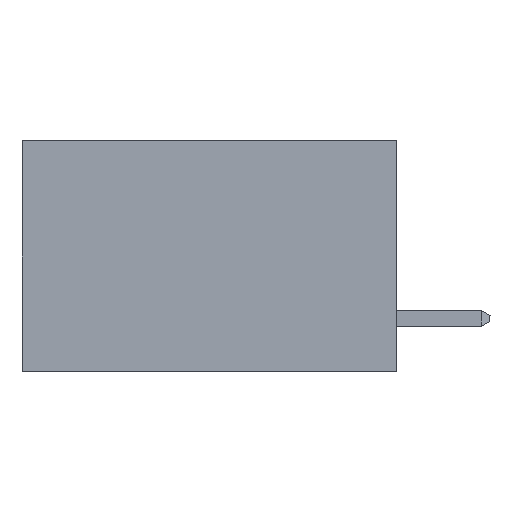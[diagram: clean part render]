
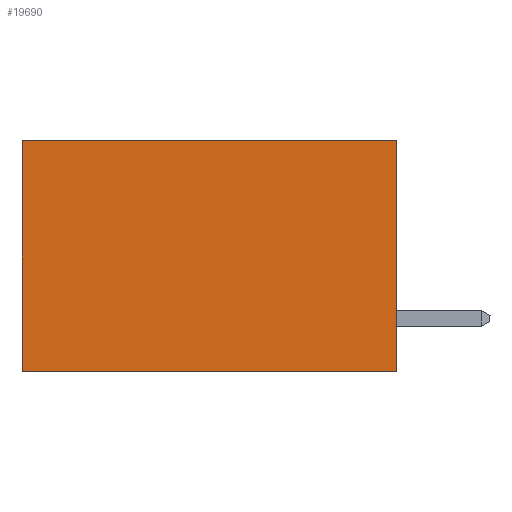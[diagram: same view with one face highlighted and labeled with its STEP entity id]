
A CAD part, left-side view. The second image highlights one B-rep face of the part: STEP entity #19690.
In plain terms, the highlighted planar face has unit normal (-1, 0, 0).
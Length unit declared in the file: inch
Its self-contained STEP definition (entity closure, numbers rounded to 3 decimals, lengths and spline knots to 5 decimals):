
#173 = DIRECTION ( 'NONE',  ( 0., 0., -1. ) ) ;
#183 = LINE ( 'NONE', #4333, #14905 ) ;
#1043 = CARTESIAN_POINT ( 'NONE',  ( 0.2615, 0.6, -0.37 ) ) ;
#1919 = ORIENTED_EDGE ( 'NONE', *, *, #18246, .T. ) ;
#2238 = AXIS2_PLACEMENT_3D ( 'NONE', #3078, #10826, #23860 ) ;
#2930 = VECTOR ( 'NONE', #15390, 39.37008 ) ;
#3078 = CARTESIAN_POINT ( 'NONE',  ( 0.2615, 0., -0.37 ) ) ;
#3537 = LINE ( 'NONE', #15925, #2930 ) ;
#3597 = VECTOR ( 'NONE', #173, 39.37008 ) ;
#4333 = CARTESIAN_POINT ( 'NONE',  ( 0.2615, 0., 0. ) ) ;
#5578 = EDGE_CURVE ( 'NONE', #16073, #18407, #3537, .T. ) ;
#6772 = CARTESIAN_POINT ( 'NONE',  ( 0.2615, 0.6, 0. ) ) ;
#7467 = VERTEX_POINT ( 'NONE', #8602 ) ;
#8249 = DIRECTION ( 'NONE',  ( 0., 1., 0. ) ) ;
#8602 = CARTESIAN_POINT ( 'NONE',  ( 0.2615, 0., 0. ) ) ;
#8747 = LINE ( 'NONE', #9761, #3597 ) ;
#9715 = FACE_OUTER_BOUND ( 'NONE', #13788, .T. ) ;
#9761 = CARTESIAN_POINT ( 'NONE',  ( 0.2615, 0., -0.37 ) ) ;
#10826 = DIRECTION ( 'NONE',  ( 1., 0., 0. ) ) ;
#11342 = ORIENTED_EDGE ( 'NONE', *, *, #11344, .T. ) ;
#11344 = EDGE_CURVE ( 'NONE', #20825, #18407, #14593, .T. ) ;
#13788 = EDGE_LOOP ( 'NONE', ( #11342, #17797, #16109, #1919 ) ) ;
#14593 = LINE ( 'NONE', #22226, #18987 ) ;
#14905 = VECTOR ( 'NONE', #8249, 39.37008 ) ;
#15390 = DIRECTION ( 'NONE',  ( 0., 1., 0. ) ) ;
#15925 = CARTESIAN_POINT ( 'NONE',  ( 0.2615, 0., -0.37 ) ) ;
#16073 = VERTEX_POINT ( 'NONE', #16374 ) ;
#16109 = ORIENTED_EDGE ( 'NONE', *, *, #21173, .F. ) ;
#16374 = CARTESIAN_POINT ( 'NONE',  ( 0.2615, 0., -0.37 ) ) ;
#17797 = ORIENTED_EDGE ( 'NONE', *, *, #5578, .F. ) ;
#18246 = EDGE_CURVE ( 'NONE', #7467, #20825, #183, .T. ) ;
#18407 = VERTEX_POINT ( 'NONE', #1043 ) ;
#18987 = VECTOR ( 'NONE', #21725, 39.37008 ) ;
#19690 = ADVANCED_FACE ( 'NONE', ( #9715 ), #22073, .F. ) ;
#20825 = VERTEX_POINT ( 'NONE', #6772 ) ;
#21173 = EDGE_CURVE ( 'NONE', #7467, #16073, #8747, .T. ) ;
#21725 = DIRECTION ( 'NONE',  ( 0., 0., -1. ) ) ;
#22073 = PLANE ( 'NONE',  #2238 ) ;
#22226 = CARTESIAN_POINT ( 'NONE',  ( 0.2615, 0.6, -0.37 ) ) ;
#23860 = DIRECTION ( 'NONE',  ( 0., 0., -1. ) ) ;
